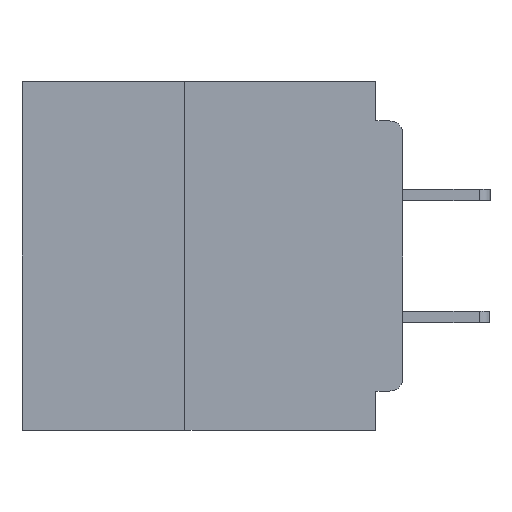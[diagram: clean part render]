
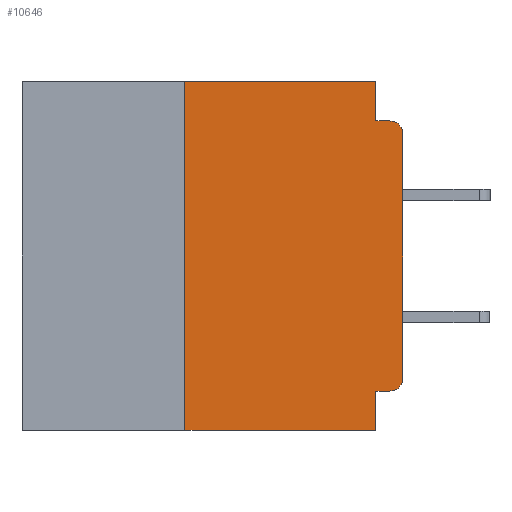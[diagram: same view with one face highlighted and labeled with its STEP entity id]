
A CAD part, left-side view. The second image highlights one B-rep face of the part: STEP entity #10646.
In plain terms, the highlighted planar face has unit normal (-1, 0, 0).
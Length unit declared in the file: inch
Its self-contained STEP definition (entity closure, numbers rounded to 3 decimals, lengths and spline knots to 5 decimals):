
#120 = LINE ( 'NONE', #3734, #7727 ) ;
#464 = VERTEX_POINT ( 'NONE', #26819 ) ;
#652 = ORIENTED_EDGE ( 'NONE', *, *, #6440, .T. ) ;
#1622 = DIRECTION ( 'NONE',  ( 0., 0., -1. ) ) ;
#3734 = CARTESIAN_POINT ( 'NONE',  ( 0., 0.437, 0. ) ) ;
#3869 = DIRECTION ( 'NONE',  ( 0., -1., 0. ) ) ;
#3880 = LINE ( 'NONE', #3971, #36990 ) ;
#3971 = CARTESIAN_POINT ( 'NONE',  ( 0., 0.031, -0.4 ) ) ;
#4012 = VERTEX_POINT ( 'NONE', #23404 ) ;
#4065 = DIRECTION ( 'NONE',  ( 0., 1., 0. ) ) ;
#4687 = LINE ( 'NONE', #10351, #29296 ) ;
#5009 = EDGE_CURVE ( 'NONE', #36588, #8308, #120, .T. ) ;
#5618 = DIRECTION ( 'NONE',  ( -1., 0., 0. ) ) ;
#6440 = EDGE_CURVE ( 'NONE', #28713, #12172, #9085, .T. ) ;
#6694 = CARTESIAN_POINT ( 'NONE',  ( 0., 0.437, -0.4 ) ) ;
#6838 = DIRECTION ( 'NONE',  ( 0., -1., 0. ) ) ;
#7267 = DIRECTION ( 'NONE',  ( -1., 0., 0. ) ) ;
#7727 = VECTOR ( 'NONE', #3869, 39.37008 ) ;
#7898 = ORIENTED_EDGE ( 'NONE', *, *, #34892, .F. ) ;
#8004 = PLANE ( 'NONE',  #37890 ) ;
#8308 = VERTEX_POINT ( 'NONE', #20354 ) ;
#9085 = LINE ( 'NONE', #6694, #25123 ) ;
#9696 = VERTEX_POINT ( 'NONE', #25299 ) ;
#10351 = CARTESIAN_POINT ( 'NONE',  ( 0., 0.031, 0. ) ) ;
#10500 = EDGE_CURVE ( 'NONE', #464, #4012, #21717, .T. ) ;
#10646 = ADVANCED_FACE ( 'NONE', ( #24227 ), #8004, .F. ) ;
#11282 = CARTESIAN_POINT ( 'NONE',  ( 0., 0.437, 0. ) ) ;
#11633 = DIRECTION ( 'NONE',  ( 0., 0., 1. ) ) ;
#12172 = VERTEX_POINT ( 'NONE', #19191 ) ;
#13282 = VECTOR ( 'NONE', #4065, 39.37008 ) ;
#13401 = ORIENTED_EDGE ( 'NONE', *, *, #37048, .T. ) ;
#13684 = ORIENTED_EDGE ( 'NONE', *, *, #17047, .F. ) ;
#14892 = CARTESIAN_POINT ( 'NONE',  ( 0., 0.031, -0.045 ) ) ;
#14936 = CARTESIAN_POINT ( 'NONE',  ( 0., 0.015, -0.045 ) ) ;
#15208 = VECTOR ( 'NONE', #19828, 39.37008 ) ;
#15493 = ORIENTED_EDGE ( 'NONE', *, *, #23110, .F. ) ;
#15614 = LINE ( 'NONE', #33957, #40054 ) ;
#16175 = LINE ( 'NONE', #29394, #15208 ) ;
#16323 = AXIS2_PLACEMENT_3D ( 'NONE', #24837, #5618, #28058 ) ;
#16352 = ORIENTED_EDGE ( 'NONE', *, *, #23953, .T. ) ;
#16929 = DIRECTION ( 'NONE',  ( 0., 0., -1. ) ) ;
#17047 = EDGE_CURVE ( 'NONE', #41423, #38588, #16175, .T. ) ;
#18673 = CARTESIAN_POINT ( 'NONE',  ( 0., 0.25, -0.4 ) ) ;
#19168 = VERTEX_POINT ( 'NONE', #32135 ) ;
#19191 = CARTESIAN_POINT ( 'NONE',  ( 0., 0.031, -0.4 ) ) ;
#19828 = DIRECTION ( 'NONE',  ( 0., -1., 0. ) ) ;
#20048 = CARTESIAN_POINT ( 'NONE',  ( 0., 0., -0.355 ) ) ;
#20354 = CARTESIAN_POINT ( 'NONE',  ( 0., 0.031, 0. ) ) ;
#20888 = DIRECTION ( 'NONE',  ( 1., 0., 0. ) ) ;
#21717 = LINE ( 'NONE', #20048, #13282 ) ;
#22059 = EDGE_LOOP ( 'NONE', ( #35602, #16352, #13684, #7898, #36685, #39111, #652, #15493, #22501, #13401 ) ) ;
#22501 = ORIENTED_EDGE ( 'NONE', *, *, #10500, .F. ) ;
#22920 = CARTESIAN_POINT ( 'NONE',  ( 0., 0., 0. ) ) ;
#23110 = EDGE_CURVE ( 'NONE', #4012, #12172, #3880, .T. ) ;
#23404 = CARTESIAN_POINT ( 'NONE',  ( 0., 0.031, -0.355 ) ) ;
#23953 = EDGE_CURVE ( 'NONE', #19168, #38588, #30455, .T. ) ;
#24155 = EDGE_CURVE ( 'NONE', #9696, #19168, #24417, .T. ) ;
#24227 = FACE_OUTER_BOUND ( 'NONE', #22059, .T. ) ;
#24417 = LINE ( 'NONE', #22920, #31933 ) ;
#24837 = CARTESIAN_POINT ( 'NONE',  ( 0., 0.015, -0.06 ) ) ;
#25123 = VECTOR ( 'NONE', #6838, 39.37008 ) ;
#25299 = CARTESIAN_POINT ( 'NONE',  ( 0., 0., -0.34 ) ) ;
#26479 = CARTESIAN_POINT ( 'NONE',  ( 0., 0.015, -0.34 ) ) ;
#26819 = CARTESIAN_POINT ( 'NONE',  ( 0., 0.015, -0.355 ) ) ;
#27361 = CARTESIAN_POINT ( 'NONE',  ( 0., 0.25, 0. ) ) ;
#28058 = DIRECTION ( 'NONE',  ( 0., 0., -1. ) ) ;
#28713 = VERTEX_POINT ( 'NONE', #18673 ) ;
#29296 = VECTOR ( 'NONE', #29499, 39.37008 ) ;
#29394 = CARTESIAN_POINT ( 'NONE',  ( 0., 0., -0.045 ) ) ;
#29499 = DIRECTION ( 'NONE',  ( 0., 0., -1. ) ) ;
#29694 = DIRECTION ( 'NONE',  ( 0., 0., -1. ) ) ;
#30455 = CIRCLE ( 'NONE', #16323, 0.015 ) ;
#31136 = CIRCLE ( 'NONE', #32513, 0.015 ) ;
#31933 = VECTOR ( 'NONE', #38972, 39.37008 ) ;
#32135 = CARTESIAN_POINT ( 'NONE',  ( 0., 0., -0.06 ) ) ;
#32513 = AXIS2_PLACEMENT_3D ( 'NONE', #26479, #7267, #29694 ) ;
#33957 = CARTESIAN_POINT ( 'NONE',  ( 0., 0.25, -0.4 ) ) ;
#34892 = EDGE_CURVE ( 'NONE', #8308, #41423, #4687, .T. ) ;
#35602 = ORIENTED_EDGE ( 'NONE', *, *, #24155, .T. ) ;
#36588 = VERTEX_POINT ( 'NONE', #27361 ) ;
#36685 = ORIENTED_EDGE ( 'NONE', *, *, #5009, .F. ) ;
#36990 = VECTOR ( 'NONE', #16929, 39.37008 ) ;
#37048 = EDGE_CURVE ( 'NONE', #464, #9696, #31136, .T. ) ;
#37844 = EDGE_CURVE ( 'NONE', #28713, #36588, #15614, .T. ) ;
#37890 = AXIS2_PLACEMENT_3D ( 'NONE', #11282, #20888, #1622 ) ;
#38588 = VERTEX_POINT ( 'NONE', #14936 ) ;
#38972 = DIRECTION ( 'NONE',  ( 0., 0., 1. ) ) ;
#39111 = ORIENTED_EDGE ( 'NONE', *, *, #37844, .F. ) ;
#40054 = VECTOR ( 'NONE', #11633, 39.37008 ) ;
#41423 = VERTEX_POINT ( 'NONE', #14892 ) ;
